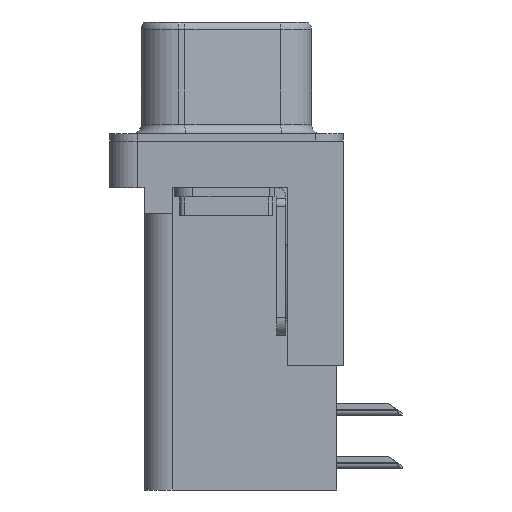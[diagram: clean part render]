
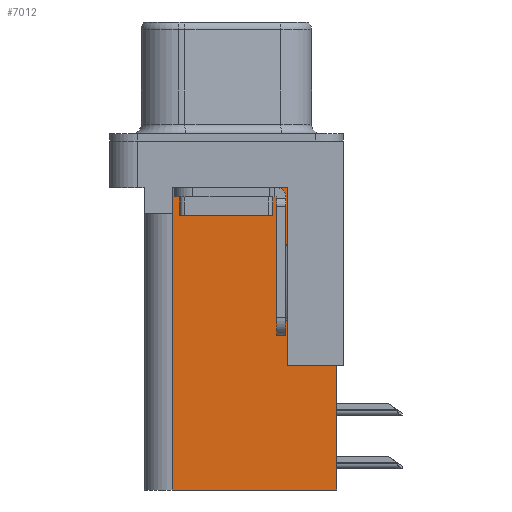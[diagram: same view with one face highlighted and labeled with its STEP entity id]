
A CAD part, left-side view. The second image highlights one B-rep face of the part: STEP entity #7012.
In plain terms, the highlighted planar face has unit normal (-1, 0, 0).
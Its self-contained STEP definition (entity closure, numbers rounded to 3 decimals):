
#493 = VECTOR ( 'NONE', #17442, 1000. ) ;
#904 = CARTESIAN_POINT ( 'NONE',  ( 3.79, -3.295, -12.05 ) ) ;
#952 = DIRECTION ( 'NONE',  ( 1., 0., 0. ) ) ;
#1179 = LINE ( 'NONE', #3605, #13836 ) ;
#1244 = LINE ( 'NONE', #12937, #493 ) ;
#1332 = EDGE_LOOP ( 'NONE', ( #21470, #23672, #8123, #11972, #18185, #20794, #25034, #8638 ) ) ;
#2685 = CARTESIAN_POINT ( 'NONE',  ( 3.79, 0., -3.9 ) ) ;
#3012 = DIRECTION ( 'NONE',  ( 0., 1., 0. ) ) ;
#3184 = FACE_OUTER_BOUND ( 'NONE', #1332, .T. ) ;
#3310 = DIRECTION ( 'NONE',  ( 0., 1., 0. ) ) ;
#3391 = LINE ( 'NONE', #2685, #26083 ) ;
#3605 = CARTESIAN_POINT ( 'NONE',  ( 3.79, -5.925, -2. ) ) ;
#4092 = LINE ( 'NONE', #23245, #20430 ) ;
#4379 = VECTOR ( 'NONE', #3012, 1000. ) ;
#5151 = VECTOR ( 'NONE', #24250, 1000. ) ;
#5319 = LINE ( 'NONE', #5761, #27845 ) ;
#5761 = CARTESIAN_POINT ( 'NONE',  ( 3.79, 2.895, -3.9 ) ) ;
#5929 = DIRECTION ( 'NONE',  ( 0., 0., -1. ) ) ;
#7012 = ADVANCED_FACE ( 'NONE', ( #3184 ), #25230, .F. ) ;
#7287 = CARTESIAN_POINT ( 'NONE',  ( 3.79, 2.925, -3.9 ) ) ;
#8123 = ORIENTED_EDGE ( 'NONE', *, *, #26973, .T. ) ;
#8562 = VERTEX_POINT ( 'NONE', #12669 ) ;
#8608 = VERTEX_POINT ( 'NONE', #12862 ) ;
#8638 = ORIENTED_EDGE ( 'NONE', *, *, #10410, .T. ) ;
#8979 = CARTESIAN_POINT ( 'NONE',  ( 3.79, -6.295, -12.05 ) ) ;
#9175 = EDGE_CURVE ( 'NONE', #23735, #22538, #1244, .T. ) ;
#9522 = DIRECTION ( 'NONE',  ( 0., 1., 0. ) ) ;
#9716 = VECTOR ( 'NONE', #24329, 1000. ) ;
#9965 = CARTESIAN_POINT ( 'NONE',  ( 3.79, 2.895, -3.9 ) ) ;
#10086 = EDGE_CURVE ( 'NONE', #8562, #23735, #4092, .T. ) ;
#10214 = EDGE_CURVE ( 'NONE', #8608, #8562, #1179, .T. ) ;
#10379 = EDGE_CURVE ( 'NONE', #8608, #27983, #16271, .T. ) ;
#10410 = EDGE_CURVE ( 'NONE', #27983, #12439, #22104, .T. ) ;
#11972 = ORIENTED_EDGE ( 'NONE', *, *, #9175, .F. ) ;
#12174 = CARTESIAN_POINT ( 'NONE',  ( 3.79, -3.295, -18.76 ) ) ;
#12439 = VERTEX_POINT ( 'NONE', #17095 ) ;
#12669 = CARTESIAN_POINT ( 'NONE',  ( 3.79, -5.925, -18.76 ) ) ;
#12862 = CARTESIAN_POINT ( 'NONE',  ( 3.79, -5.925, -12.05 ) ) ;
#12937 = CARTESIAN_POINT ( 'NONE',  ( 3.79, 2.925, -18.76 ) ) ;
#13306 = CARTESIAN_POINT ( 'NONE',  ( 3.79, 2.895, -2.5 ) ) ;
#13373 = CARTESIAN_POINT ( 'NONE',  ( 3.79, -3.295, -18.76 ) ) ;
#13836 = VECTOR ( 'NONE', #5929, 1000. ) ;
#14425 = VERTEX_POINT ( 'NONE', #9965 ) ;
#16255 = AXIS2_PLACEMENT_3D ( 'NONE', #12174, #952, #16650 ) ;
#16271 = LINE ( 'NONE', #8979, #5151 ) ;
#16650 = DIRECTION ( 'NONE',  ( 0., 1., 0. ) ) ;
#17095 = CARTESIAN_POINT ( 'NONE',  ( 3.79, -3.295, -2.5 ) ) ;
#17442 = DIRECTION ( 'NONE',  ( 0., 0., 1. ) ) ;
#18185 = ORIENTED_EDGE ( 'NONE', *, *, #10086, .F. ) ;
#18353 = VERTEX_POINT ( 'NONE', #13306 ) ;
#18634 = CARTESIAN_POINT ( 'NONE',  ( 3.79, -3.295, -2.5 ) ) ;
#20430 = VECTOR ( 'NONE', #3310, 1000. ) ;
#20794 = ORIENTED_EDGE ( 'NONE', *, *, #10214, .F. ) ;
#21447 = CARTESIAN_POINT ( 'NONE',  ( 3.79, 2.925, -18.76 ) ) ;
#21470 = ORIENTED_EDGE ( 'NONE', *, *, #21989, .T. ) ;
#21989 = EDGE_CURVE ( 'NONE', #12439, #18353, #26982, .T. ) ;
#22104 = LINE ( 'NONE', #13373, #9716 ) ;
#22538 = VERTEX_POINT ( 'NONE', #7287 ) ;
#23245 = CARTESIAN_POINT ( 'NONE',  ( 3.79, -3.295, -18.76 ) ) ;
#23672 = ORIENTED_EDGE ( 'NONE', *, *, #24672, .T. ) ;
#23735 = VERTEX_POINT ( 'NONE', #21447 ) ;
#24250 = DIRECTION ( 'NONE',  ( 0., 1., 0. ) ) ;
#24329 = DIRECTION ( 'NONE',  ( 0., 0., 1. ) ) ;
#24672 = EDGE_CURVE ( 'NONE', #18353, #14425, #5319, .T. ) ;
#25034 = ORIENTED_EDGE ( 'NONE', *, *, #10379, .T. ) ;
#25230 = PLANE ( 'NONE',  #16255 ) ;
#26083 = VECTOR ( 'NONE', #9522, 1000. ) ;
#26973 = EDGE_CURVE ( 'NONE', #14425, #22538, #3391, .T. ) ;
#26982 = LINE ( 'NONE', #18634, #4379 ) ;
#27779 = DIRECTION ( 'NONE',  ( 0., 0., -1. ) ) ;
#27845 = VECTOR ( 'NONE', #27779, 1000. ) ;
#27983 = VERTEX_POINT ( 'NONE', #904 ) ;
